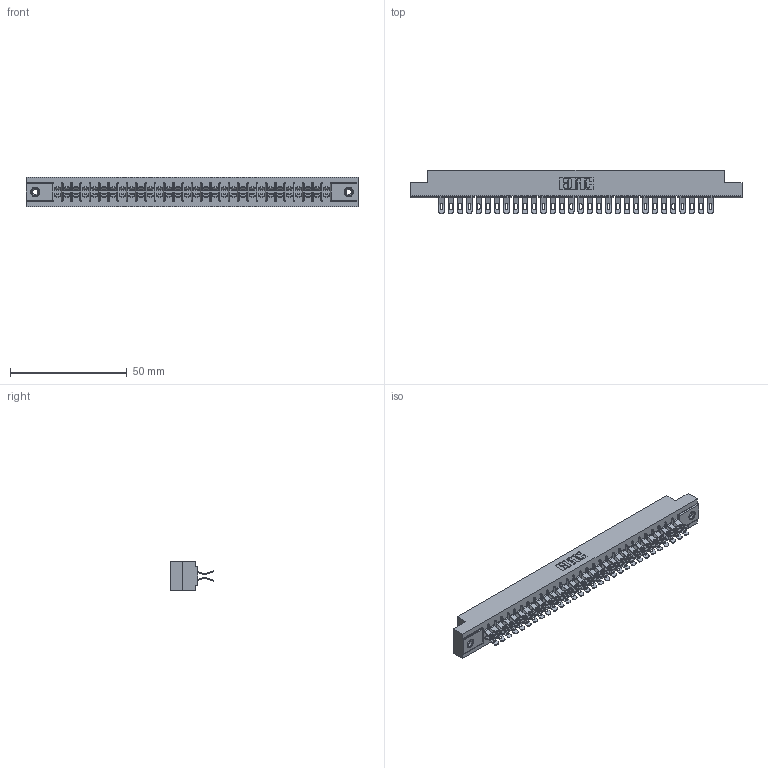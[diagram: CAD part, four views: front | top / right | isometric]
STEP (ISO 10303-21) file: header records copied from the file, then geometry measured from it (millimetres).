
FILE_DESCRIPTION (( 'STEP AP203' ), '1' );
FILE_NAME ('305-060-555-208.STEP', '2019-09-10T01:20:20', ( '' ), ( '' ), 'SwSTEP 2.0', 'SolidWorks 2016', '' );
FILE_SCHEMA (( 'CONFIG_CONTROL_DESIGN' ));
Length unit declared in the file: inch
Products named in the file (4): 345-250-001_345-250-003-102; 305-060-555-208; 305 Part_.156 Dia; 305-290-001_555
Assembly tree (63 placements, depth 2):
  305-060-555-208
    305 Part_.156 Dia
    305-290-001_555  x60
    345-250-001_345-250-003-102  x2
Bounding box: 141.88 x 18.41 x 12.7 mm (x, y, z)
Volume: 14896.4 mm3; surface area: 19835.2 mm2
Topology: 63 solids, 63 shells, 4136 faces, 12302 edges, 8032 vertices
Faces by surface type: plane 2020, cylinder 1980, sphere 120, cone 12, torus 4
Entity records: 35752 total; most frequent: CARTESIAN_POINT 5917, ORIENTED_EDGE 5856, DIRECTION 5738, EDGE_CURVE 2928, LINE 2332, VECTOR 2332, VERTEX_POINT 1866, AXIS2_PLACEMENT_3D 1703
